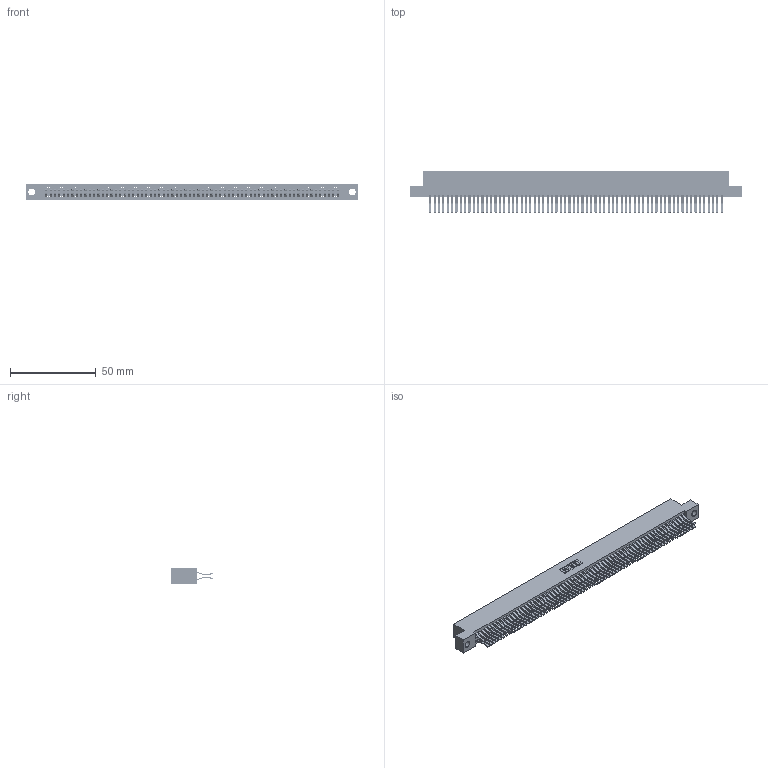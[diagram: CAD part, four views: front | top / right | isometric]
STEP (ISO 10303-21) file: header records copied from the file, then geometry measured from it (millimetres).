
FILE_DESCRIPTION (( 'STEP AP203' ), '1' );
FILE_NAME ('395-136-560-204.STEP', '2021-06-18T03:11:47', ( '' ), ( '' ), 'SwSTEP 2.0', 'SolidWorks 2020', '' );
FILE_SCHEMA (( 'CONFIG_CONTROL_DESIGN' ));
Length unit declared in the file: inch
Products named in the file (3): 345-292-001_560 Tail; 395-136-560-204; 345 Part_Flush Mounting Lugs - 0.156 Dia-TI
Assembly tree (137 placements, depth 2):
  395-136-560-204
    345 Part_Flush Mounting Lugs - 0.156 Dia-TI
    345-292-001_560 Tail  x136
Bounding box: 193.93 x 24.45 x 9.4 mm (x, y, z)
Volume: 19865.3 mm3; surface area: 32012 mm2
Topology: 137 solids, 137 shells, 7212 faces, 21457 edges, 14122 vertices
Faces by surface type: plane 4582, cylinder 2630
Entity records: 50361 total; most frequent: CARTESIAN_POINT 8422, ORIENTED_EDGE 8354, DIRECTION 7397, EDGE_CURVE 4177, VECTOR 3769, LINE 3769, VERTEX_POINT 2782, AXIS2_PLACEMENT_3D 1814
